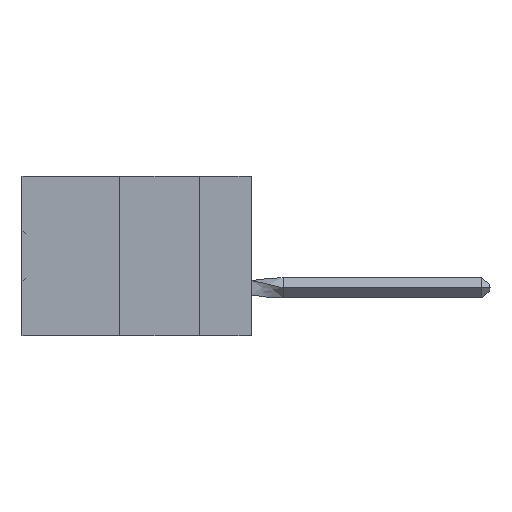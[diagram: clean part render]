
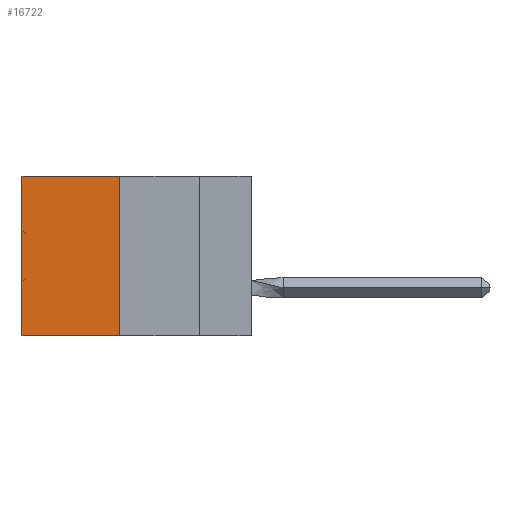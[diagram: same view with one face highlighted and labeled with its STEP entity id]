
A CAD part, left-side view. The second image highlights one B-rep face of the part: STEP entity #16722.
In plain terms, the highlighted planar face has unit normal (-1, 0, 0).
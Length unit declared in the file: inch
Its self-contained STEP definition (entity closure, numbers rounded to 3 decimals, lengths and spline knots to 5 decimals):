
#1040 = EDGE_CURVE ( 'NONE', #55793, #56440, #34666, .T. ) ;
#1572 = DIRECTION ( 'NONE',  ( 0., 0., -1. ) ) ;
#2861 = CARTESIAN_POINT ( 'NONE',  ( 0.305, 0.72, -0.5 ) ) ;
#4602 = DIRECTION ( 'NONE',  ( 0., 1., 0. ) ) ;
#5078 = LINE ( 'NONE', #34950, #50369 ) ;
#5146 = VECTOR ( 'NONE', #54542, 39.37008 ) ;
#11724 = CARTESIAN_POINT ( 'NONE',  ( 0.305, 0.72, 0. ) ) ;
#12344 = EDGE_CURVE ( 'NONE', #21199, #55793, #27146, .T. ) ;
#12353 = DIRECTION ( 'NONE',  ( 0., 0., -1. ) ) ;
#14445 = ORIENTED_EDGE ( 'NONE', *, *, #15867, .T. ) ;
#15393 = LINE ( 'NONE', #24049, #40079 ) ;
#15867 = EDGE_CURVE ( 'NONE', #21199, #56554, #5078, .T. ) ;
#16485 = CARTESIAN_POINT ( 'NONE',  ( 0.305, 0.413, -0.5 ) ) ;
#16722 = ADVANCED_FACE ( 'NONE', ( #34784 ), #25613, .F. ) ;
#19420 = CARTESIAN_POINT ( 'NONE',  ( 0.305, 0.413, -0.5 ) ) ;
#21199 = VERTEX_POINT ( 'NONE', #37168 ) ;
#21381 = ORIENTED_EDGE ( 'NONE', *, *, #40134, .T. ) ;
#23144 = ORIENTED_EDGE ( 'NONE', *, *, #12344, .F. ) ;
#24049 = CARTESIAN_POINT ( 'NONE',  ( 0.305, 0.72, -0.5 ) ) ;
#25613 = PLANE ( 'NONE',  #27449 ) ;
#27146 = LINE ( 'NONE', #19420, #5146 ) ;
#27449 = AXIS2_PLACEMENT_3D ( 'NONE', #48208, #38593, #12353 ) ;
#34666 = LINE ( 'NONE', #16485, #46310 ) ;
#34784 = FACE_OUTER_BOUND ( 'NONE', #35055, .T. ) ;
#34950 = CARTESIAN_POINT ( 'NONE',  ( 0.305, 0.413, 0. ) ) ;
#35055 = EDGE_LOOP ( 'NONE', ( #21381, #36584, #23144, #14445 ) ) ;
#36584 = ORIENTED_EDGE ( 'NONE', *, *, #1040, .F. ) ;
#37168 = CARTESIAN_POINT ( 'NONE',  ( 0.305, 0.413, 0. ) ) ;
#38593 = DIRECTION ( 'NONE',  ( 1., 0., 0. ) ) ;
#40079 = VECTOR ( 'NONE', #1572, 39.37008 ) ;
#40134 = EDGE_CURVE ( 'NONE', #56554, #56440, #15393, .T. ) ;
#46310 = VECTOR ( 'NONE', #50833, 39.37008 ) ;
#47881 = CARTESIAN_POINT ( 'NONE',  ( 0.305, 0.413, -0.5 ) ) ;
#48208 = CARTESIAN_POINT ( 'NONE',  ( 0.305, 0.413, -0.5 ) ) ;
#50369 = VECTOR ( 'NONE', #4602, 39.37008 ) ;
#50833 = DIRECTION ( 'NONE',  ( 0., 1., 0. ) ) ;
#54542 = DIRECTION ( 'NONE',  ( 0., 0., -1. ) ) ;
#55793 = VERTEX_POINT ( 'NONE', #47881 ) ;
#56440 = VERTEX_POINT ( 'NONE', #2861 ) ;
#56554 = VERTEX_POINT ( 'NONE', #11724 ) ;
